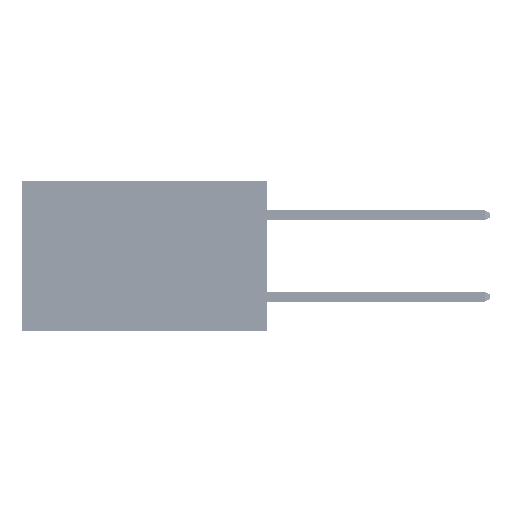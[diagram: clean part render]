
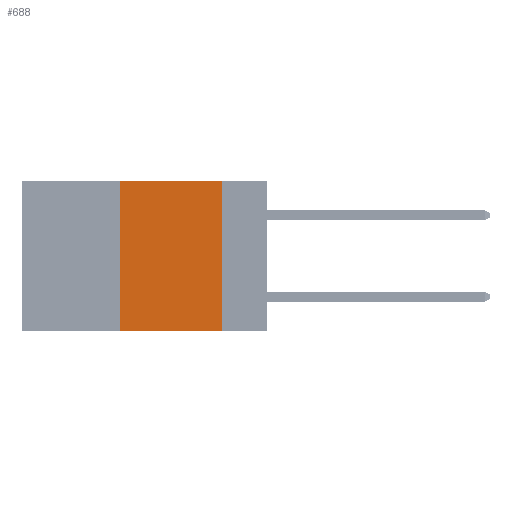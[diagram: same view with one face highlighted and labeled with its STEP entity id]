
A CAD part, left-side view. The second image highlights one B-rep face of the part: STEP entity #688.
In plain terms, the highlighted planar face has unit normal (-1, 0, 0).
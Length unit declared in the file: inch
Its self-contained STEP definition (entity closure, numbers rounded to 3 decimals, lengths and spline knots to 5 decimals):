
#688 = ADVANCED_FACE ( 'NONE', ( #14148 ), #28883, .F. ) ;
#4975 = CARTESIAN_POINT ( 'NONE',  ( 0., 0.36, 0. ) ) ;
#5537 = AXIS2_PLACEMENT_3D ( 'NONE', #27571, #43977, #28732 ) ;
#6427 = ORIENTED_EDGE ( 'NONE', *, *, #28921, .T. ) ;
#8185 = VERTEX_POINT ( 'NONE', #36803 ) ;
#8265 = VERTEX_POINT ( 'NONE', #15142 ) ;
#11600 = VECTOR ( 'NONE', #12782, 39.37008 ) ;
#12782 = DIRECTION ( 'NONE',  ( 0., 0., 1. ) ) ;
#14148 = FACE_OUTER_BOUND ( 'NONE', #45893, .T. ) ;
#15142 = CARTESIAN_POINT ( 'NONE',  ( 0., 0.36, -0.37 ) ) ;
#18443 = LINE ( 'NONE', #33225, #33938 ) ;
#19394 = LINE ( 'NONE', #23209, #37317 ) ;
#20492 = LINE ( 'NONE', #4975, #11600 ) ;
#23209 = CARTESIAN_POINT ( 'NONE',  ( 0., 0.6, 0. ) ) ;
#23785 = EDGE_CURVE ( 'NONE', #38881, #36006, #19394, .T. ) ;
#26746 = EDGE_CURVE ( 'NONE', #8265, #38881, #20492, .T. ) ;
#27571 = CARTESIAN_POINT ( 'NONE',  ( 0., 0.6, 0. ) ) ;
#27877 = CARTESIAN_POINT ( 'NONE',  ( 0., 0.11, 0. ) ) ;
#28732 = DIRECTION ( 'NONE',  ( 0., 0., -1. ) ) ;
#28883 = PLANE ( 'NONE',  #5537 ) ;
#28921 = EDGE_CURVE ( 'NONE', #8265, #8185, #18443, .T. ) ;
#33225 = CARTESIAN_POINT ( 'NONE',  ( 0., 0.6, -0.37 ) ) ;
#33938 = VECTOR ( 'NONE', #45142, 39.37008 ) ;
#34881 = VECTOR ( 'NONE', #44653, 39.37008 ) ;
#36006 = VERTEX_POINT ( 'NONE', #27877 ) ;
#36803 = CARTESIAN_POINT ( 'NONE',  ( 0., 0.11, -0.37 ) ) ;
#37296 = LINE ( 'NONE', #48001, #34881 ) ;
#37317 = VECTOR ( 'NONE', #38091, 39.37008 ) ;
#38091 = DIRECTION ( 'NONE',  ( 0., -1., 0. ) ) ;
#38881 = VERTEX_POINT ( 'NONE', #48909 ) ;
#41724 = EDGE_CURVE ( 'NONE', #36006, #8185, #37296, .T. ) ;
#43977 = DIRECTION ( 'NONE',  ( 1., 0., 0. ) ) ;
#44212 = ORIENTED_EDGE ( 'NONE', *, *, #41724, .F. ) ;
#44653 = DIRECTION ( 'NONE',  ( 0., 0., -1. ) ) ;
#44656 = ORIENTED_EDGE ( 'NONE', *, *, #23785, .F. ) ;
#44764 = ORIENTED_EDGE ( 'NONE', *, *, #26746, .F. ) ;
#45142 = DIRECTION ( 'NONE',  ( 0., -1., 0. ) ) ;
#45893 = EDGE_LOOP ( 'NONE', ( #44212, #44656, #44764, #6427 ) ) ;
#48001 = CARTESIAN_POINT ( 'NONE',  ( 0., 0.11, 0. ) ) ;
#48909 = CARTESIAN_POINT ( 'NONE',  ( 0., 0.36, 0. ) ) ;
